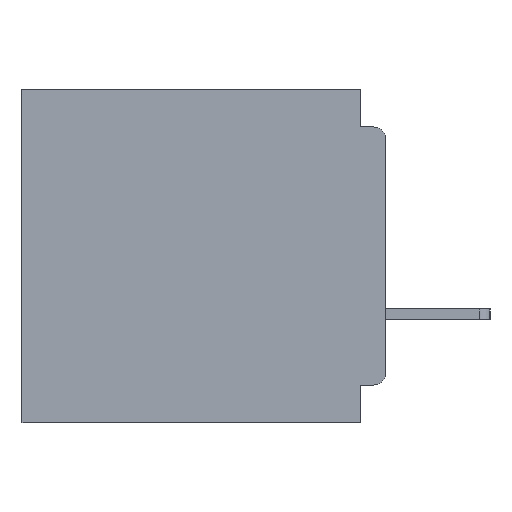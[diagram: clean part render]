
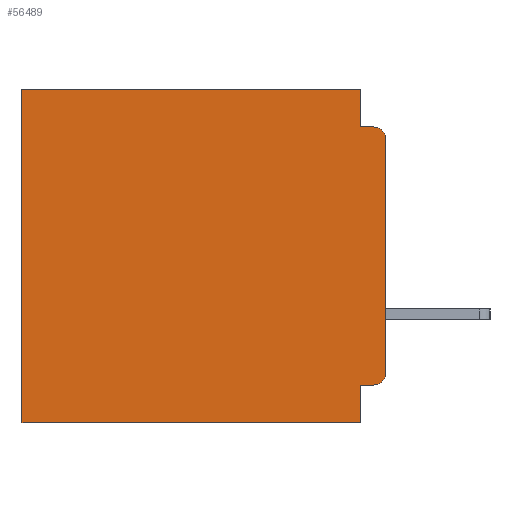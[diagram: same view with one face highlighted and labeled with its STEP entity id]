
A CAD part, left-side view. The second image highlights one B-rep face of the part: STEP entity #56489.
In plain terms, the highlighted planar face has unit normal (-1, 0, 0).
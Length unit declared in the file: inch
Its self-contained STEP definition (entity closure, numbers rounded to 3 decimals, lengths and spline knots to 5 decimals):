
#246 = CARTESIAN_POINT ( 'NONE',  ( 0.3, 0., -0.4 ) ) ;
#392 = EDGE_CURVE ( 'NONE', #51865, #1239, #6314, .T. ) ;
#1069 = VECTOR ( 'NONE', #21433, 39.37008 ) ;
#1131 = ORIENTED_EDGE ( 'NONE', *, *, #8181, .F. ) ;
#1239 = VERTEX_POINT ( 'NONE', #30445 ) ;
#1514 = ORIENTED_EDGE ( 'NONE', *, *, #392, .T. ) ;
#4841 = EDGE_CURVE ( 'NONE', #51865, #43419, #39946, .T. ) ;
#4909 = AXIS2_PLACEMENT_3D ( 'NONE', #20166, #50611, #24559 ) ;
#5113 = FACE_OUTER_BOUND ( 'NONE', #8266, .T. ) ;
#6314 = CIRCLE ( 'NONE', #17467, 0.015 ) ;
#7768 = LINE ( 'NONE', #49867, #18064 ) ;
#8181 = EDGE_CURVE ( 'NONE', #17098, #55107, #48859, .T. ) ;
#8266 = EDGE_LOOP ( 'NONE', ( #12384, #12469, #1131, #43493, #33954, #29452, #15515, #55520, #16301, #1514 ) ) ;
#10294 = AXIS2_PLACEMENT_3D ( 'NONE', #29698, #42777, #16719 ) ;
#11385 = LINE ( 'NONE', #21829, #44740 ) ;
#12384 = ORIENTED_EDGE ( 'NONE', *, *, #15793, .F. ) ;
#12469 = ORIENTED_EDGE ( 'NONE', *, *, #32519, .T. ) ;
#12888 = DIRECTION ( 'NONE',  ( 0., 0., -1. ) ) ;
#13114 = CARTESIAN_POINT ( 'NONE',  ( 0.3, 0.437, 0. ) ) ;
#15448 = VECTOR ( 'NONE', #42044, 39.37008 ) ;
#15515 = ORIENTED_EDGE ( 'NONE', *, *, #22533, .F. ) ;
#15693 = CARTESIAN_POINT ( 'NONE',  ( 0.3, 0.031, 0. ) ) ;
#15793 = EDGE_CURVE ( 'NONE', #46203, #1239, #21661, .T. ) ;
#16301 = ORIENTED_EDGE ( 'NONE', *, *, #4841, .F. ) ;
#16719 = DIRECTION ( 'NONE',  ( 0., 0., -1. ) ) ;
#17098 = VERTEX_POINT ( 'NONE', #53539 ) ;
#17169 = CARTESIAN_POINT ( 'NONE',  ( 0.3, 0.031, -0.355 ) ) ;
#17250 = EDGE_CURVE ( 'NONE', #37754, #34840, #35073, .T. ) ;
#17467 = AXIS2_PLACEMENT_3D ( 'NONE', #31270, #49874, #47141 ) ;
#17621 = DIRECTION ( 'NONE',  ( 0., 1., 0. ) ) ;
#18064 = VECTOR ( 'NONE', #45468, 39.37008 ) ;
#18983 = VERTEX_POINT ( 'NONE', #19365 ) ;
#19365 = CARTESIAN_POINT ( 'NONE',  ( 0.3, 0.031, -0.4 ) ) ;
#19420 = VECTOR ( 'NONE', #28810, 39.37008 ) ;
#20166 = CARTESIAN_POINT ( 'NONE',  ( 0.3, 0.015, -0.06 ) ) ;
#21433 = DIRECTION ( 'NONE',  ( 0., -1., 0. ) ) ;
#21661 = LINE ( 'NONE', #246, #31896 ) ;
#21829 = CARTESIAN_POINT ( 'NONE',  ( 0.3, 0., -0.4 ) ) ;
#22533 = EDGE_CURVE ( 'NONE', #18983, #28427, #11385, .T. ) ;
#24448 = CARTESIAN_POINT ( 'NONE',  ( 0.3, 0., 0. ) ) ;
#24559 = DIRECTION ( 'NONE',  ( 0., 0., -1. ) ) ;
#27592 = CARTESIAN_POINT ( 'NONE',  ( 0.3, 0.031, -0.4 ) ) ;
#28427 = VERTEX_POINT ( 'NONE', #44099 ) ;
#28810 = DIRECTION ( 'NONE',  ( 0., 1., 0. ) ) ;
#29246 = EDGE_CURVE ( 'NONE', #43419, #18983, #51567, .T. ) ;
#29452 = ORIENTED_EDGE ( 'NONE', *, *, #30519, .T. ) ;
#29698 = CARTESIAN_POINT ( 'NONE',  ( 0.3, 0., -0.4 ) ) ;
#30235 = CARTESIAN_POINT ( 'NONE',  ( 0.3, 0.031, 0. ) ) ;
#30445 = CARTESIAN_POINT ( 'NONE',  ( 0.3, 0., -0.34 ) ) ;
#30519 = EDGE_CURVE ( 'NONE', #34840, #28427, #7768, .T. ) ;
#31270 = CARTESIAN_POINT ( 'NONE',  ( 0.3, 0.015, -0.34 ) ) ;
#31896 = VECTOR ( 'NONE', #43752, 39.37008 ) ;
#32519 = EDGE_CURVE ( 'NONE', #46203, #55107, #39670, .T. ) ;
#32766 = LINE ( 'NONE', #30235, #55802 ) ;
#33954 = ORIENTED_EDGE ( 'NONE', *, *, #17250, .T. ) ;
#34840 = VERTEX_POINT ( 'NONE', #13114 ) ;
#35073 = LINE ( 'NONE', #24448, #19420 ) ;
#37060 = CARTESIAN_POINT ( 'NONE',  ( 0.3, 0.015, -0.355 ) ) ;
#37754 = VERTEX_POINT ( 'NONE', #15693 ) ;
#38167 = CARTESIAN_POINT ( 'NONE',  ( 0.3, 0., -0.06 ) ) ;
#38405 = PLANE ( 'NONE',  #10294 ) ;
#39670 = CIRCLE ( 'NONE', #4909, 0.015 ) ;
#39946 = LINE ( 'NONE', #47832, #15448 ) ;
#39996 = VECTOR ( 'NONE', #45025, 39.37008 ) ;
#42044 = DIRECTION ( 'NONE',  ( 0., 1., 0. ) ) ;
#42777 = DIRECTION ( 'NONE',  ( 1., 0., 0. ) ) ;
#43419 = VERTEX_POINT ( 'NONE', #17169 ) ;
#43493 = ORIENTED_EDGE ( 'NONE', *, *, #53885, .F. ) ;
#43752 = DIRECTION ( 'NONE',  ( 0., 0., -1. ) ) ;
#44099 = CARTESIAN_POINT ( 'NONE',  ( 0.3, 0.437, -0.4 ) ) ;
#44740 = VECTOR ( 'NONE', #17621, 39.37008 ) ;
#45025 = DIRECTION ( 'NONE',  ( 0., 0., -1. ) ) ;
#45468 = DIRECTION ( 'NONE',  ( 0., 0., -1. ) ) ;
#46203 = VERTEX_POINT ( 'NONE', #38167 ) ;
#47141 = DIRECTION ( 'NONE',  ( 0., 0., -1. ) ) ;
#47832 = CARTESIAN_POINT ( 'NONE',  ( 0.3, 0., -0.355 ) ) ;
#48859 = LINE ( 'NONE', #51847, #1069 ) ;
#49867 = CARTESIAN_POINT ( 'NONE',  ( 0.3, 0.437, -0.4 ) ) ;
#49874 = DIRECTION ( 'NONE',  ( -1., 0., 0. ) ) ;
#50611 = DIRECTION ( 'NONE',  ( -1., 0., 0. ) ) ;
#51567 = LINE ( 'NONE', #27592, #39996 ) ;
#51847 = CARTESIAN_POINT ( 'NONE',  ( 0.3, 0., -0.045 ) ) ;
#51865 = VERTEX_POINT ( 'NONE', #37060 ) ;
#53539 = CARTESIAN_POINT ( 'NONE',  ( 0.3, 0.031, -0.045 ) ) ;
#53885 = EDGE_CURVE ( 'NONE', #37754, #17098, #32766, .T. ) ;
#54143 = CARTESIAN_POINT ( 'NONE',  ( 0.3, 0.015, -0.045 ) ) ;
#55107 = VERTEX_POINT ( 'NONE', #54143 ) ;
#55520 = ORIENTED_EDGE ( 'NONE', *, *, #29246, .F. ) ;
#55802 = VECTOR ( 'NONE', #12888, 39.37008 ) ;
#56489 = ADVANCED_FACE ( 'NONE', ( #5113 ), #38405, .F. ) ;
